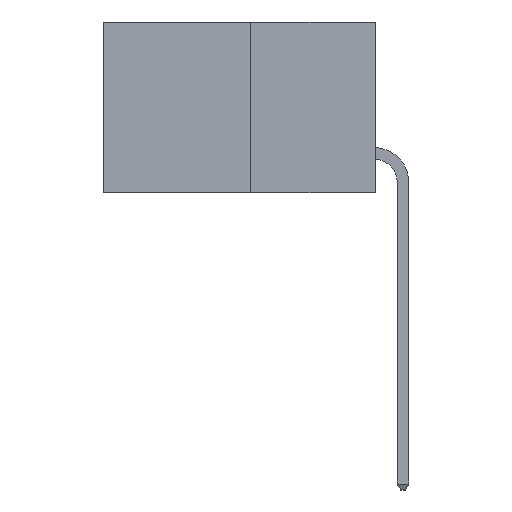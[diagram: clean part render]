
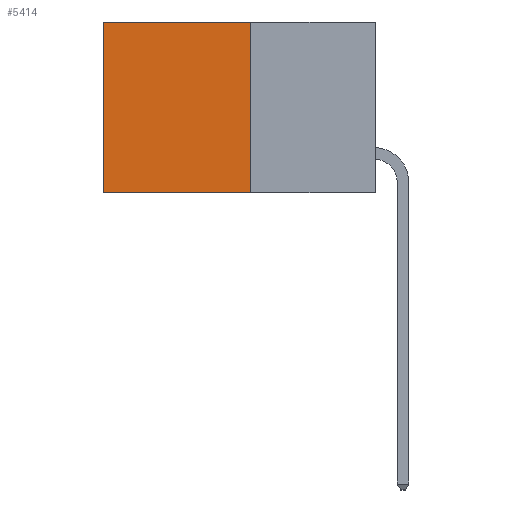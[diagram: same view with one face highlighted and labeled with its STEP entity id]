
A CAD part, left-side view. The second image highlights one B-rep face of the part: STEP entity #5414.
In plain terms, the highlighted planar face has unit normal (-1, 0, 0).
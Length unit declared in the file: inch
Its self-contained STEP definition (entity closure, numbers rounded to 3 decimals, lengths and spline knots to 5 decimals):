
#432 = AXIS2_PLACEMENT_3D ( 'NONE', #2030, #8203, #4253 ) ;
#497 = VERTEX_POINT ( 'NONE', #549 ) ;
#549 = CARTESIAN_POINT ( 'NONE',  ( 0.277, 0.27, -0.37 ) ) ;
#551 = VERTEX_POINT ( 'NONE', #7616 ) ;
#891 = FACE_OUTER_BOUND ( 'NONE', #4645, .T. ) ;
#1296 = VERTEX_POINT ( 'NONE', #8266 ) ;
#1378 = EDGE_CURVE ( 'NONE', #1296, #497, #3873, .T. ) ;
#1409 = VECTOR ( 'NONE', #2033, 39.37008 ) ;
#1798 = LINE ( 'NONE', #6475, #5468 ) ;
#2030 = CARTESIAN_POINT ( 'NONE',  ( 0.277, 0.27, -0.37 ) ) ;
#2033 = DIRECTION ( 'NONE',  ( 0., 0., -1. ) ) ;
#2621 = ORIENTED_EDGE ( 'NONE', *, *, #6861, .F. ) ;
#3643 = ORIENTED_EDGE ( 'NONE', *, *, #6207, .T. ) ;
#3798 = CARTESIAN_POINT ( 'NONE',  ( 0.277, 0.27, -0.37 ) ) ;
#3873 = LINE ( 'NONE', #4421, #1409 ) ;
#3878 = CARTESIAN_POINT ( 'NONE',  ( 0.277, 0.59, 0. ) ) ;
#4253 = DIRECTION ( 'NONE',  ( 0., 0., -1. ) ) ;
#4421 = CARTESIAN_POINT ( 'NONE',  ( 0.277, 0.27, -0.37 ) ) ;
#4571 = ORIENTED_EDGE ( 'NONE', *, *, #8921, .T. ) ;
#4645 = EDGE_LOOP ( 'NONE', ( #3643, #2621, #6456, #4571 ) ) ;
#5151 = DIRECTION ( 'NONE',  ( 0., 0., -1. ) ) ;
#5284 = DIRECTION ( 'NONE',  ( 0., 1., 0. ) ) ;
#5414 = ADVANCED_FACE ( 'NONE', ( #891 ), #5648, .F. ) ;
#5468 = VECTOR ( 'NONE', #5151, 39.37008 ) ;
#5566 = LINE ( 'NONE', #3798, #7119 ) ;
#5648 = PLANE ( 'NONE',  #432 ) ;
#5759 = VERTEX_POINT ( 'NONE', #3878 ) ;
#6207 = EDGE_CURVE ( 'NONE', #5759, #551, #1798, .T. ) ;
#6456 = ORIENTED_EDGE ( 'NONE', *, *, #1378, .F. ) ;
#6475 = CARTESIAN_POINT ( 'NONE',  ( 0.277, 0.59, -0.37 ) ) ;
#6861 = EDGE_CURVE ( 'NONE', #497, #551, #5566, .T. ) ;
#7119 = VECTOR ( 'NONE', #8373, 39.37008 ) ;
#7180 = LINE ( 'NONE', #8489, #8591 ) ;
#7616 = CARTESIAN_POINT ( 'NONE',  ( 0.277, 0.59, -0.37 ) ) ;
#8203 = DIRECTION ( 'NONE',  ( 1., 0., 0. ) ) ;
#8266 = CARTESIAN_POINT ( 'NONE',  ( 0.277, 0.27, 0. ) ) ;
#8373 = DIRECTION ( 'NONE',  ( 0., 1., 0. ) ) ;
#8489 = CARTESIAN_POINT ( 'NONE',  ( 0.277, 0.27, 0. ) ) ;
#8591 = VECTOR ( 'NONE', #5284, 39.37008 ) ;
#8921 = EDGE_CURVE ( 'NONE', #1296, #5759, #7180, .T. ) ;
